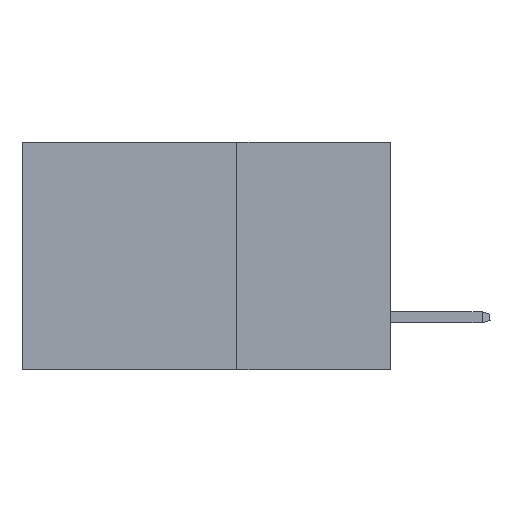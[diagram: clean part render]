
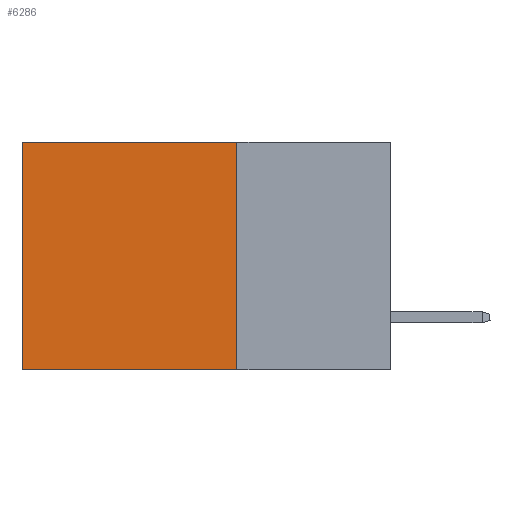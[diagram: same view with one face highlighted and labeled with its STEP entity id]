
A CAD part, left-side view. The second image highlights one B-rep face of the part: STEP entity #6286.
In plain terms, the highlighted planar face has unit normal (-1, 0, 0).
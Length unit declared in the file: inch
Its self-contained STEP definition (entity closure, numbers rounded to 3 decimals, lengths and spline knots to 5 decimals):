
#422 = VECTOR ( 'NONE', #22604, 39.37008 ) ;
#1771 = CARTESIAN_POINT ( 'NONE',  ( 0.2875, 0.6, -0.37 ) ) ;
#2123 = ORIENTED_EDGE ( 'NONE', *, *, #4527, .T. ) ;
#2131 = CARTESIAN_POINT ( 'NONE',  ( 0.2875, 0.25, 0. ) ) ;
#2828 = DIRECTION ( 'NONE',  ( 0., 0., -1. ) ) ;
#3051 = VECTOR ( 'NONE', #18321, 39.37008 ) ;
#3296 = AXIS2_PLACEMENT_3D ( 'NONE', #2131, #8918, #2828 ) ;
#4078 = CARTESIAN_POINT ( 'NONE',  ( 0.2875, 0.6, 0. ) ) ;
#4527 = EDGE_CURVE ( 'NONE', #25590, #10801, #23293, .T. ) ;
#5340 = ORIENTED_EDGE ( 'NONE', *, *, #19693, .T. ) ;
#6265 = ORIENTED_EDGE ( 'NONE', *, *, #18660, .F. ) ;
#6286 = ADVANCED_FACE ( 'NONE', ( #25800 ), #25160, .F. ) ;
#7416 = EDGE_CURVE ( 'NONE', #8509, #10801, #9345, .T. ) ;
#8509 = VERTEX_POINT ( 'NONE', #15534 ) ;
#8872 = DIRECTION ( 'NONE',  ( 0., 1., 0. ) ) ;
#8918 = DIRECTION ( 'NONE',  ( 1., 0., 0. ) ) ;
#9345 = LINE ( 'NONE', #23305, #25156 ) ;
#9852 = CARTESIAN_POINT ( 'NONE',  ( 0.2875, 0.25, 0. ) ) ;
#9962 = CARTESIAN_POINT ( 'NONE',  ( 0.2875, 0.25, 0. ) ) ;
#10801 = VERTEX_POINT ( 'NONE', #1771 ) ;
#12545 = EDGE_LOOP ( 'NONE', ( #2123, #18631, #6265, #5340 ) ) ;
#12851 = LINE ( 'NONE', #25371, #21249 ) ;
#15534 = CARTESIAN_POINT ( 'NONE',  ( 0.2875, 0.25, -0.37 ) ) ;
#18298 = CARTESIAN_POINT ( 'NONE',  ( 0.2875, 0.6, 0. ) ) ;
#18321 = DIRECTION ( 'NONE',  ( 0., 0., -1. ) ) ;
#18631 = ORIENTED_EDGE ( 'NONE', *, *, #7416, .F. ) ;
#18660 = EDGE_CURVE ( 'NONE', #21239, #8509, #20439, .T. ) ;
#19693 = EDGE_CURVE ( 'NONE', #21239, #25590, #12851, .T. ) ;
#20439 = LINE ( 'NONE', #9852, #3051 ) ;
#21239 = VERTEX_POINT ( 'NONE', #9962 ) ;
#21249 = VECTOR ( 'NONE', #8872, 39.37008 ) ;
#22604 = DIRECTION ( 'NONE',  ( 0., 0., -1. ) ) ;
#23293 = LINE ( 'NONE', #4078, #422 ) ;
#23305 = CARTESIAN_POINT ( 'NONE',  ( 0.2875, 0.25, -0.37 ) ) ;
#25156 = VECTOR ( 'NONE', #25213, 39.37008 ) ;
#25160 = PLANE ( 'NONE',  #3296 ) ;
#25213 = DIRECTION ( 'NONE',  ( 0., 1., 0. ) ) ;
#25371 = CARTESIAN_POINT ( 'NONE',  ( 0.2875, 0.25, 0. ) ) ;
#25590 = VERTEX_POINT ( 'NONE', #18298 ) ;
#25800 = FACE_OUTER_BOUND ( 'NONE', #12545, .T. ) ;
